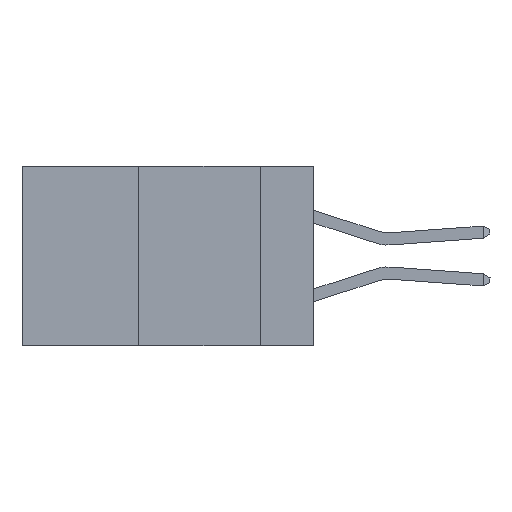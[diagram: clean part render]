
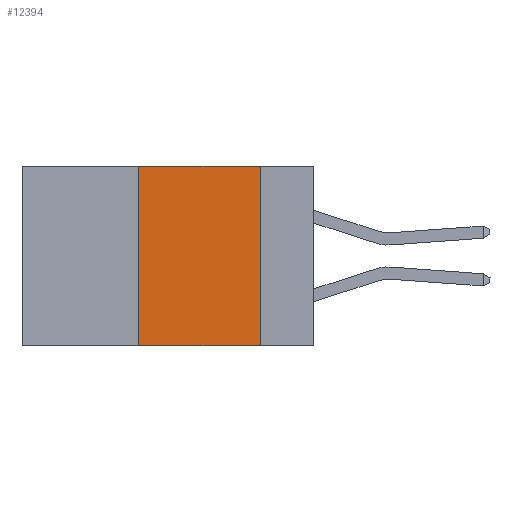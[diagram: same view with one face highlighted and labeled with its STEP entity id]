
A CAD part, left-side view. The second image highlights one B-rep face of the part: STEP entity #12394.
In plain terms, the highlighted planar face has unit normal (-1, 0, 0).
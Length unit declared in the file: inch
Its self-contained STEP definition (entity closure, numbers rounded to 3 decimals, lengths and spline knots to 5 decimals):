
#73 = EDGE_CURVE ( 'NONE', #1621, #6641, #12843, .T. ) ;
#1322 = DIRECTION ( 'NONE',  ( 0., 0., -1. ) ) ;
#1621 = VERTEX_POINT ( 'NONE', #19739 ) ;
#2301 = CARTESIAN_POINT ( 'NONE',  ( 0., 0.36, 0. ) ) ;
#2582 = DIRECTION ( 'NONE',  ( 0., 0., 1. ) ) ;
#3937 = EDGE_LOOP ( 'NONE', ( #4440, #6203, #21679, #12578 ) ) ;
#4440 = ORIENTED_EDGE ( 'NONE', *, *, #10091, .F. ) ;
#5389 = DIRECTION ( 'NONE',  ( 0., -1., 0. ) ) ;
#6203 = ORIENTED_EDGE ( 'NONE', *, *, #10998, .F. ) ;
#6641 = VERTEX_POINT ( 'NONE', #21085 ) ;
#6659 = CARTESIAN_POINT ( 'NONE',  ( 0., 0.6, 0. ) ) ;
#6922 = PLANE ( 'NONE',  #23184 ) ;
#7188 = VERTEX_POINT ( 'NONE', #17643 ) ;
#7190 = CARTESIAN_POINT ( 'NONE',  ( 0., 0.11, -0.37 ) ) ;
#8070 = EDGE_CURVE ( 'NONE', #1621, #21129, #14383, .T. ) ;
#8202 = VECTOR ( 'NONE', #12238, 39.37008 ) ;
#8240 = VECTOR ( 'NONE', #11385, 39.37008 ) ;
#10065 = VECTOR ( 'NONE', #5389, 39.37008 ) ;
#10091 = EDGE_CURVE ( 'NONE', #7188, #21129, #12591, .T. ) ;
#10998 = EDGE_CURVE ( 'NONE', #6641, #7188, #17951, .T. ) ;
#11385 = DIRECTION ( 'NONE',  ( 0., 0., -1. ) ) ;
#12238 = DIRECTION ( 'NONE',  ( 0., -1., 0. ) ) ;
#12394 = ADVANCED_FACE ( 'NONE', ( #17723 ), #6922, .F. ) ;
#12498 = DIRECTION ( 'NONE',  ( 1., 0., 0. ) ) ;
#12578 = ORIENTED_EDGE ( 'NONE', *, *, #8070, .T. ) ;
#12591 = LINE ( 'NONE', #22302, #8240 ) ;
#12843 = LINE ( 'NONE', #2301, #17114 ) ;
#14253 = CARTESIAN_POINT ( 'NONE',  ( 0., 0.6, 0. ) ) ;
#14383 = LINE ( 'NONE', #14595, #10065 ) ;
#14595 = CARTESIAN_POINT ( 'NONE',  ( 0., 0.6, -0.37 ) ) ;
#17114 = VECTOR ( 'NONE', #2582, 39.37008 ) ;
#17643 = CARTESIAN_POINT ( 'NONE',  ( 0., 0.11, 0. ) ) ;
#17723 = FACE_OUTER_BOUND ( 'NONE', #3937, .T. ) ;
#17951 = LINE ( 'NONE', #6659, #8202 ) ;
#19739 = CARTESIAN_POINT ( 'NONE',  ( 0., 0.36, -0.37 ) ) ;
#21085 = CARTESIAN_POINT ( 'NONE',  ( 0., 0.36, 0. ) ) ;
#21129 = VERTEX_POINT ( 'NONE', #7190 ) ;
#21679 = ORIENTED_EDGE ( 'NONE', *, *, #73, .F. ) ;
#22302 = CARTESIAN_POINT ( 'NONE',  ( 0., 0.11, 0. ) ) ;
#23184 = AXIS2_PLACEMENT_3D ( 'NONE', #14253, #12498, #1322 ) ;
